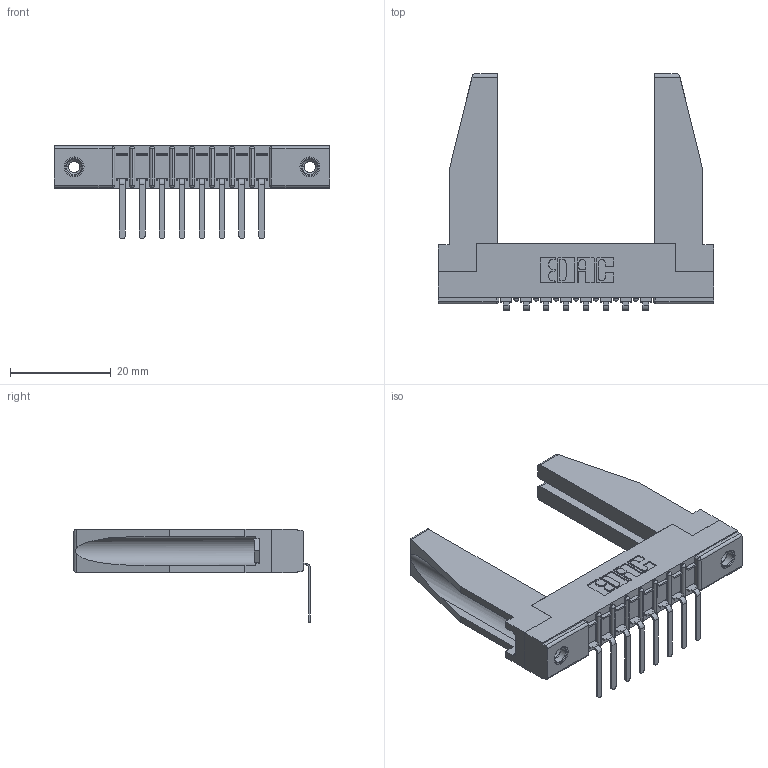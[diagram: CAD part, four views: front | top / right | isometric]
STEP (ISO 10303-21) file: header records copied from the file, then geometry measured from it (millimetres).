
FILE_DESCRIPTION (( 'STEP AP203' ), '1' );
FILE_NAME ('357-008-557-178.STEP', '2019-09-16T17:55:11', ( '' ), ( '' ), 'SwSTEP 2.0', 'SolidWorks 2016', '' );
FILE_SCHEMA (( 'CONFIG_CONTROL_DESIGN' ));
Length unit declared in the file: inch
Products named in the file (5): 307 Part_.156 Dia Mounting Holes; 345-250-001_345-250-001-102; 307-290-002_557; 357-008-557-178; 307-220-078
Assembly tree (13 placements, depth 2):
  357-008-557-178
    307 Part_.156 Dia Mounting Holes
    307-290-002_557  x8
    307-220-078  x2
    345-250-001_345-250-001-102  x2
Bounding box: 54.71 x 47.03 x 18.67 mm (x, y, z)
Volume: 7619.5 mm3; surface area: 9769.7 mm2
Topology: 13 solids, 13 shells, 881 faces, 2605 edges, 1702 vertices
Faces by surface type: plane 530, cylinder 317, sphere 18, cone 12, torus 4
Entity records: 14343 total; most frequent: CARTESIAN_POINT 2414, ORIENTED_EDGE 2360, DIRECTION 2318, EDGE_CURVE 1180, LINE 890, VECTOR 890, VERTEX_POINT 768, AXIS2_PLACEMENT_3D 714
